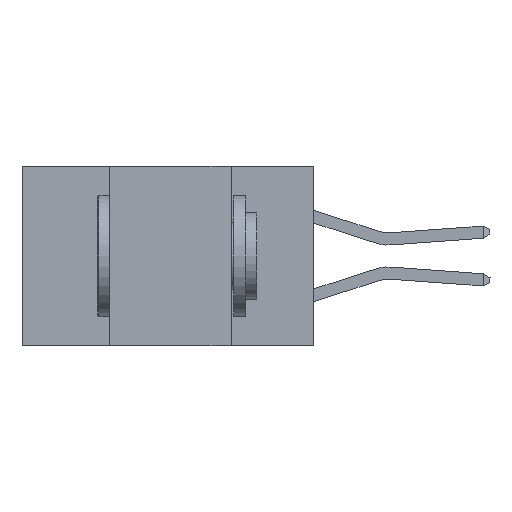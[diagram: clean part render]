
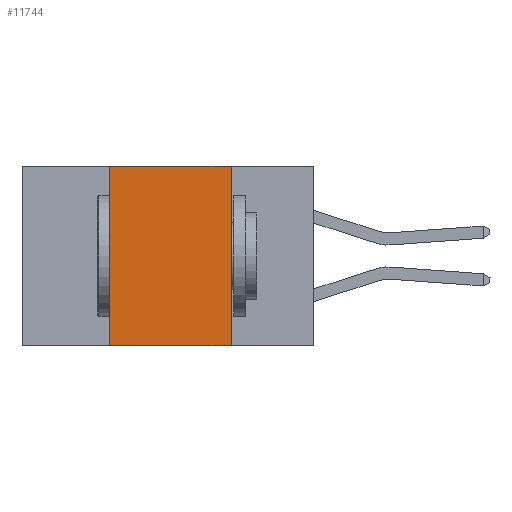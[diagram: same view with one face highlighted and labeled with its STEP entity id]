
A CAD part, left-side view. The second image highlights one B-rep face of the part: STEP entity #11744.
In plain terms, the highlighted planar face has unit normal (-1, 0, 0).
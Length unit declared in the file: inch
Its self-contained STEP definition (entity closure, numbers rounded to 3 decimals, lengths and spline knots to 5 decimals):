
#609 = DIRECTION ( 'NONE',  ( 0., 0., -1. ) ) ;
#1241 = AXIS2_PLACEMENT_3D ( 'NONE', #11178, #19419, #609 ) ;
#1581 = LINE ( 'NONE', #8368, #14862 ) ;
#1810 = DIRECTION ( 'NONE',  ( 0., -1., 0. ) ) ;
#2468 = CARTESIAN_POINT ( 'NONE',  ( 0., 0.42, -0.37 ) ) ;
#2711 = LINE ( 'NONE', #16609, #16419 ) ;
#5906 = CARTESIAN_POINT ( 'NONE',  ( 0., 0.17, -0.37 ) ) ;
#6261 = EDGE_CURVE ( 'NONE', #31269, #22111, #13766, .T. ) ;
#8368 = CARTESIAN_POINT ( 'NONE',  ( 0., 0.42, 0. ) ) ;
#9905 = EDGE_CURVE ( 'NONE', #15039, #22111, #26691, .T. ) ;
#10676 = DIRECTION ( 'NONE',  ( 0., -1., 0. ) ) ;
#10991 = EDGE_LOOP ( 'NONE', ( #24824, #14224, #19875, #14672 ) ) ;
#11178 = CARTESIAN_POINT ( 'NONE',  ( 0., 0.6, 0. ) ) ;
#11744 = ADVANCED_FACE ( 'NONE', ( #32398 ), #21654, .F. ) ;
#13766 = LINE ( 'NONE', #30876, #30844 ) ;
#14224 = ORIENTED_EDGE ( 'NONE', *, *, #21023, .F. ) ;
#14672 = ORIENTED_EDGE ( 'NONE', *, *, #6261, .T. ) ;
#14862 = VECTOR ( 'NONE', #27233, 39.37008 ) ;
#15039 = VERTEX_POINT ( 'NONE', #16696 ) ;
#16419 = VECTOR ( 'NONE', #10676, 39.37008 ) ;
#16609 = CARTESIAN_POINT ( 'NONE',  ( 0., 0.6, 0. ) ) ;
#16696 = CARTESIAN_POINT ( 'NONE',  ( 0., 0.17, 0. ) ) ;
#19419 = DIRECTION ( 'NONE',  ( 1., 0., 0. ) ) ;
#19875 = ORIENTED_EDGE ( 'NONE', *, *, #33978, .F. ) ;
#21023 = EDGE_CURVE ( 'NONE', #32045, #15039, #2711, .T. ) ;
#21654 = PLANE ( 'NONE',  #1241 ) ;
#21664 = VECTOR ( 'NONE', #33365, 39.37008 ) ;
#22111 = VERTEX_POINT ( 'NONE', #5906 ) ;
#22330 = CARTESIAN_POINT ( 'NONE',  ( 0., 0.42, 0. ) ) ;
#24824 = ORIENTED_EDGE ( 'NONE', *, *, #9905, .F. ) ;
#26691 = LINE ( 'NONE', #33601, #21664 ) ;
#27233 = DIRECTION ( 'NONE',  ( 0., 0., 1. ) ) ;
#30844 = VECTOR ( 'NONE', #1810, 39.37008 ) ;
#30876 = CARTESIAN_POINT ( 'NONE',  ( 0., 0.6, -0.37 ) ) ;
#31269 = VERTEX_POINT ( 'NONE', #2468 ) ;
#32045 = VERTEX_POINT ( 'NONE', #22330 ) ;
#32398 = FACE_OUTER_BOUND ( 'NONE', #10991, .T. ) ;
#33365 = DIRECTION ( 'NONE',  ( 0., 0., -1. ) ) ;
#33601 = CARTESIAN_POINT ( 'NONE',  ( 0., 0.17, 0. ) ) ;
#33978 = EDGE_CURVE ( 'NONE', #31269, #32045, #1581, .T. ) ;
